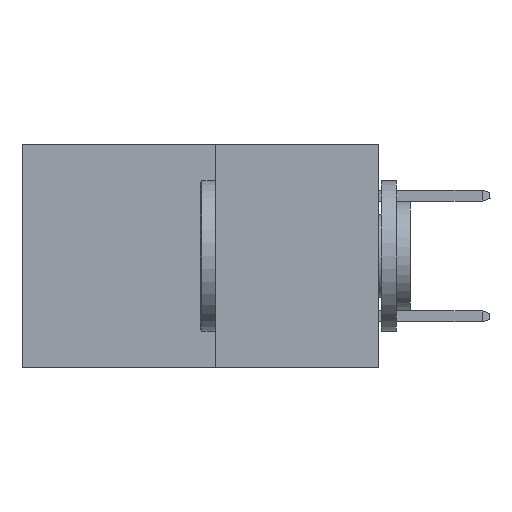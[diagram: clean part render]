
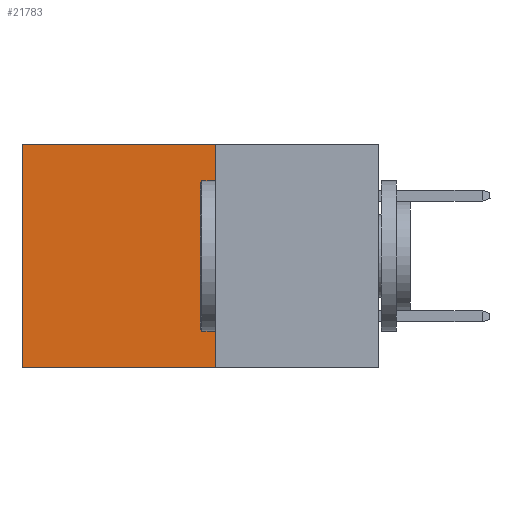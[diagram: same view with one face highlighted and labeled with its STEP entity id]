
A CAD part, left-side view. The second image highlights one B-rep face of the part: STEP entity #21783.
In plain terms, the highlighted planar face has unit normal (-1, 0, 0).
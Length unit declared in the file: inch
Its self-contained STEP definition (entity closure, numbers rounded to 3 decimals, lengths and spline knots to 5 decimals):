
#430 = DIRECTION ( 'NONE',  ( 0., 0., -1. ) ) ;
#1333 = ORIENTED_EDGE ( 'NONE', *, *, #18099, .T. ) ;
#1456 = VERTEX_POINT ( 'NONE', #11288 ) ;
#1735 = VECTOR ( 'NONE', #17756, 39.37008 ) ;
#3251 = LINE ( 'NONE', #8286, #12349 ) ;
#3465 = FACE_OUTER_BOUND ( 'NONE', #12207, .T. ) ;
#3817 = ORIENTED_EDGE ( 'NONE', *, *, #11543, .T. ) ;
#4658 = AXIS2_PLACEMENT_3D ( 'NONE', #20801, #10680, #430 ) ;
#6183 = LINE ( 'NONE', #9274, #14709 ) ;
#6321 = LINE ( 'NONE', #21047, #1735 ) ;
#7498 = CARTESIAN_POINT ( 'NONE',  ( 0.277, 0.27, 0. ) ) ;
#8286 = CARTESIAN_POINT ( 'NONE',  ( 0.277, 0.59, -0.37 ) ) ;
#8954 = PLANE ( 'NONE',  #4658 ) ;
#9274 = CARTESIAN_POINT ( 'NONE',  ( 0.277, 0.27, -0.37 ) ) ;
#10680 = DIRECTION ( 'NONE',  ( 1., 0., 0. ) ) ;
#11054 = ORIENTED_EDGE ( 'NONE', *, *, #21214, .F. ) ;
#11288 = CARTESIAN_POINT ( 'NONE',  ( 0.277, 0.59, 0. ) ) ;
#11543 = EDGE_CURVE ( 'NONE', #1456, #16624, #3251, .T. ) ;
#11987 = CARTESIAN_POINT ( 'NONE',  ( 0.277, 0.27, -0.37 ) ) ;
#12207 = EDGE_LOOP ( 'NONE', ( #3817, #13868, #11054, #1333 ) ) ;
#12349 = VECTOR ( 'NONE', #20147, 39.37008 ) ;
#12400 = VECTOR ( 'NONE', #14398, 39.37008 ) ;
#12675 = CARTESIAN_POINT ( 'NONE',  ( 0.277, 0.27, -0.37 ) ) ;
#12928 = LINE ( 'NONE', #12675, #12400 ) ;
#13868 = ORIENTED_EDGE ( 'NONE', *, *, #19373, .F. ) ;
#14398 = DIRECTION ( 'NONE',  ( 0., 1., 0. ) ) ;
#14709 = VECTOR ( 'NONE', #16124, 39.37008 ) ;
#16124 = DIRECTION ( 'NONE',  ( 0., 0., -1. ) ) ;
#16624 = VERTEX_POINT ( 'NONE', #17436 ) ;
#17436 = CARTESIAN_POINT ( 'NONE',  ( 0.277, 0.59, -0.37 ) ) ;
#17756 = DIRECTION ( 'NONE',  ( 0., 1., 0. ) ) ;
#18099 = EDGE_CURVE ( 'NONE', #21161, #1456, #6321, .T. ) ;
#19373 = EDGE_CURVE ( 'NONE', #20920, #16624, #12928, .T. ) ;
#20147 = DIRECTION ( 'NONE',  ( 0., 0., -1. ) ) ;
#20801 = CARTESIAN_POINT ( 'NONE',  ( 0.277, 0.27, -0.37 ) ) ;
#20920 = VERTEX_POINT ( 'NONE', #11987 ) ;
#21047 = CARTESIAN_POINT ( 'NONE',  ( 0.277, 0.27, 0. ) ) ;
#21161 = VERTEX_POINT ( 'NONE', #7498 ) ;
#21214 = EDGE_CURVE ( 'NONE', #21161, #20920, #6183, .T. ) ;
#21783 = ADVANCED_FACE ( 'NONE', ( #3465 ), #8954, .F. ) ;
